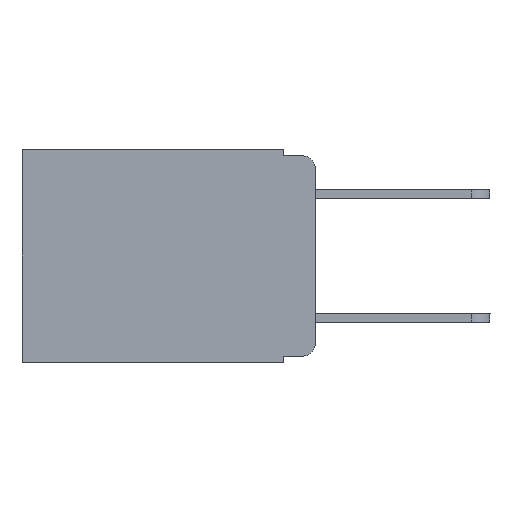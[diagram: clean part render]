
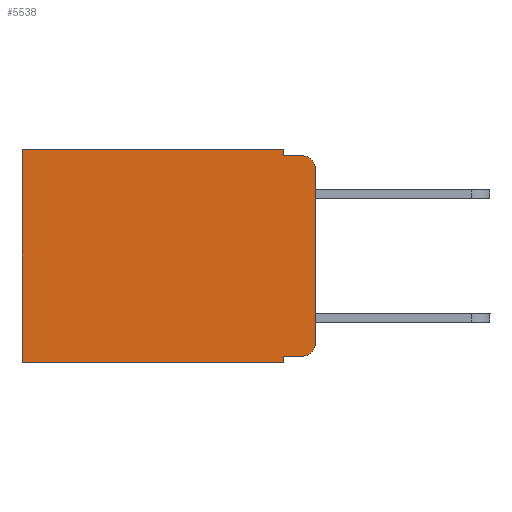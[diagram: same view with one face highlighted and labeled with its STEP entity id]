
A CAD part, left-side view. The second image highlights one B-rep face of the part: STEP entity #5538.
In plain terms, the highlighted planar face has unit normal (-1, 0, 0).
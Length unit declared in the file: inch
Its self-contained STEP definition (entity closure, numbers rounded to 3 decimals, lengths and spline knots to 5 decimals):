
#28 = DIRECTION ( 'NONE',  ( 0., 0., -1. ) ) ;
#118 = EDGE_CURVE ( 'NONE', #16784, #20428, #7919, .T. ) ;
#1105 = AXIS2_PLACEMENT_3D ( 'NONE', #3830, #5208, #10100 ) ;
#1212 = LINE ( 'NONE', #7897, #12269 ) ;
#1330 = LINE ( 'NONE', #14375, #8655 ) ;
#1684 = VECTOR ( 'NONE', #10018, 39.37008 ) ;
#2076 = EDGE_CURVE ( 'NONE', #14150, #19572, #2266, .T. ) ;
#2086 = CARTESIAN_POINT ( 'NONE',  ( 0.298, 0.02, -0.03 ) ) ;
#2182 = CARTESIAN_POINT ( 'NONE',  ( 0.298, 0.051, -0.343 ) ) ;
#2212 = VECTOR ( 'NONE', #16886, 39.37008 ) ;
#2266 = LINE ( 'NONE', #17967, #1684 ) ;
#3092 = EDGE_CURVE ( 'NONE', #16784, #4757, #3829, .T. ) ;
#3242 = DIRECTION ( 'NONE',  ( 0., 1., 0. ) ) ;
#3249 = DIRECTION ( 'NONE',  ( 0., 0., -1. ) ) ;
#3829 = CIRCLE ( 'NONE', #6523, 0.02 ) ;
#3830 = CARTESIAN_POINT ( 'NONE',  ( 0.298, 0.02, -0.313 ) ) ;
#4155 = LINE ( 'NONE', #9244, #18725 ) ;
#4564 = DIRECTION ( 'NONE',  ( 1., 0., 0. ) ) ;
#4656 = CARTESIAN_POINT ( 'NONE',  ( 0.298, 0.051, 0. ) ) ;
#4667 = EDGE_CURVE ( 'NONE', #14642, #4702, #1330, .T. ) ;
#4702 = VERTEX_POINT ( 'NONE', #16185 ) ;
#4757 = VERTEX_POINT ( 'NONE', #9513 ) ;
#5054 = DIRECTION ( 'NONE',  ( 0., 0., -1. ) ) ;
#5208 = DIRECTION ( 'NONE',  ( -1., 0., 0. ) ) ;
#5538 = ADVANCED_FACE ( 'NONE', ( #6057 ), #20506, .F. ) ;
#6057 = FACE_OUTER_BOUND ( 'NONE', #17360, .T. ) ;
#6402 = AXIS2_PLACEMENT_3D ( 'NONE', #15828, #4564, #7757 ) ;
#6523 = AXIS2_PLACEMENT_3D ( 'NONE', #2086, #8238, #5054 ) ;
#6612 = ORIENTED_EDGE ( 'NONE', *, *, #10877, .F. ) ;
#6615 = ORIENTED_EDGE ( 'NONE', *, *, #3092, .T. ) ;
#7055 = CARTESIAN_POINT ( 'NONE',  ( 0.298, 0.051, -0.333 ) ) ;
#7550 = EDGE_CURVE ( 'NONE', #14642, #9973, #11177, .T. ) ;
#7757 = DIRECTION ( 'NONE',  ( 0., 0., -1. ) ) ;
#7897 = CARTESIAN_POINT ( 'NONE',  ( 0.298, 0.473, 0. ) ) ;
#7919 = LINE ( 'NONE', #11020, #12050 ) ;
#7969 = DIRECTION ( 'NONE',  ( 0., 0., -1. ) ) ;
#8021 = CARTESIAN_POINT ( 'NONE',  ( 0.298, 0., -0.313 ) ) ;
#8139 = ORIENTED_EDGE ( 'NONE', *, *, #9008, .T. ) ;
#8238 = DIRECTION ( 'NONE',  ( -1., 0., 0. ) ) ;
#8655 = VECTOR ( 'NONE', #14583, 39.37008 ) ;
#9008 = EDGE_CURVE ( 'NONE', #4702, #20428, #18050, .T. ) ;
#9244 = CARTESIAN_POINT ( 'NONE',  ( 0.298, 0.051, -0.01 ) ) ;
#9513 = CARTESIAN_POINT ( 'NONE',  ( 0.298, 0.02, -0.01 ) ) ;
#9973 = VERTEX_POINT ( 'NONE', #2182 ) ;
#10018 = DIRECTION ( 'NONE',  ( 0., 0., -1. ) ) ;
#10100 = DIRECTION ( 'NONE',  ( 0., 0., -1. ) ) ;
#10164 = EDGE_CURVE ( 'NONE', #13935, #18806, #1212, .T. ) ;
#10877 = EDGE_CURVE ( 'NONE', #19572, #4757, #4155, .T. ) ;
#11020 = CARTESIAN_POINT ( 'NONE',  ( 0.298, 0., 0. ) ) ;
#11177 = LINE ( 'NONE', #19434, #13459 ) ;
#11994 = LINE ( 'NONE', #14881, #2212 ) ;
#12050 = VECTOR ( 'NONE', #3249, 39.37008 ) ;
#12269 = VECTOR ( 'NONE', #28, 39.37008 ) ;
#12414 = CARTESIAN_POINT ( 'NONE',  ( 0.298, 0.473, 0. ) ) ;
#12628 = CARTESIAN_POINT ( 'NONE',  ( 0.298, 0.051, -0.01 ) ) ;
#13142 = ORIENTED_EDGE ( 'NONE', *, *, #7550, .F. ) ;
#13292 = ORIENTED_EDGE ( 'NONE', *, *, #118, .F. ) ;
#13459 = VECTOR ( 'NONE', #7969, 39.37008 ) ;
#13895 = EDGE_CURVE ( 'NONE', #14150, #13935, #11994, .T. ) ;
#13935 = VERTEX_POINT ( 'NONE', #12414 ) ;
#13989 = ORIENTED_EDGE ( 'NONE', *, *, #13895, .T. ) ;
#14150 = VERTEX_POINT ( 'NONE', #4656 ) ;
#14227 = VECTOR ( 'NONE', #3242, 39.37008 ) ;
#14375 = CARTESIAN_POINT ( 'NONE',  ( 0.298, 0.051, -0.333 ) ) ;
#14532 = CARTESIAN_POINT ( 'NONE',  ( 0.298, 0.473, -0.343 ) ) ;
#14583 = DIRECTION ( 'NONE',  ( 0., -1., 0. ) ) ;
#14642 = VERTEX_POINT ( 'NONE', #7055 ) ;
#14881 = CARTESIAN_POINT ( 'NONE',  ( 0.298, 0., 0. ) ) ;
#15828 = CARTESIAN_POINT ( 'NONE',  ( 0.298, 0., 0. ) ) ;
#16078 = ORIENTED_EDGE ( 'NONE', *, *, #20490, .F. ) ;
#16185 = CARTESIAN_POINT ( 'NONE',  ( 0.298, 0.02, -0.333 ) ) ;
#16784 = VERTEX_POINT ( 'NONE', #19787 ) ;
#16886 = DIRECTION ( 'NONE',  ( 0., 1., 0. ) ) ;
#17360 = EDGE_LOOP ( 'NONE', ( #13292, #6615, #6612, #19373, #13989, #18127, #16078, #13142, #20240, #8139 ) ) ;
#17775 = LINE ( 'NONE', #19277, #14227 ) ;
#17967 = CARTESIAN_POINT ( 'NONE',  ( 0.298, 0.051, 0. ) ) ;
#18050 = CIRCLE ( 'NONE', #1105, 0.02 ) ;
#18127 = ORIENTED_EDGE ( 'NONE', *, *, #10164, .T. ) ;
#18725 = VECTOR ( 'NONE', #20501, 39.37008 ) ;
#18806 = VERTEX_POINT ( 'NONE', #14532 ) ;
#19277 = CARTESIAN_POINT ( 'NONE',  ( 0.298, 0., -0.343 ) ) ;
#19373 = ORIENTED_EDGE ( 'NONE', *, *, #2076, .F. ) ;
#19434 = CARTESIAN_POINT ( 'NONE',  ( 0.298, 0.051, 0. ) ) ;
#19572 = VERTEX_POINT ( 'NONE', #12628 ) ;
#19787 = CARTESIAN_POINT ( 'NONE',  ( 0.298, 0., -0.03 ) ) ;
#20240 = ORIENTED_EDGE ( 'NONE', *, *, #4667, .T. ) ;
#20428 = VERTEX_POINT ( 'NONE', #8021 ) ;
#20490 = EDGE_CURVE ( 'NONE', #9973, #18806, #17775, .T. ) ;
#20501 = DIRECTION ( 'NONE',  ( 0., -1., 0. ) ) ;
#20506 = PLANE ( 'NONE',  #6402 ) ;
